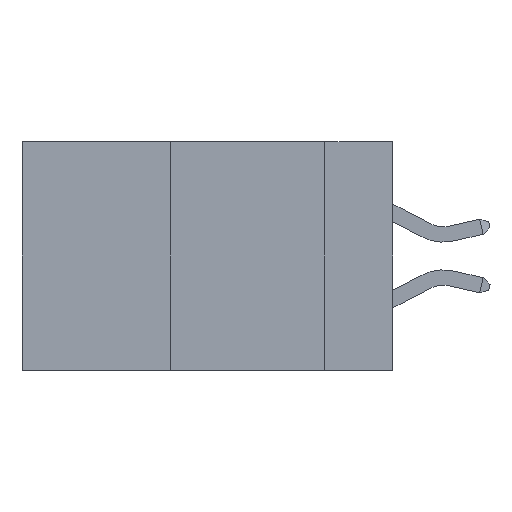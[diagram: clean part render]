
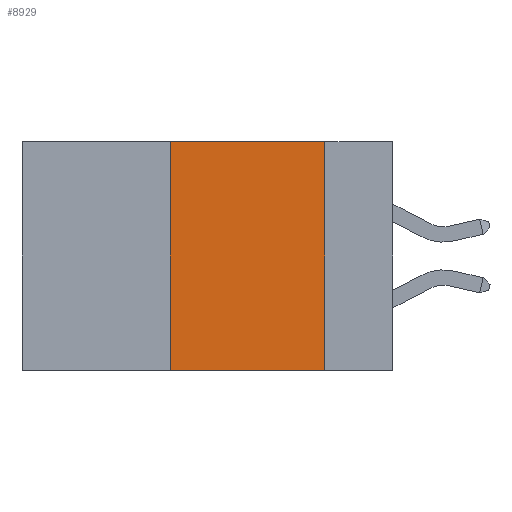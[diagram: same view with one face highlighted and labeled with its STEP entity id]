
A CAD part, left-side view. The second image highlights one B-rep face of the part: STEP entity #8929.
In plain terms, the highlighted planar face has unit normal (-1, 0, 0).
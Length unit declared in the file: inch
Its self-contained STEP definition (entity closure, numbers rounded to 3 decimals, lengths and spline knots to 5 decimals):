
#153 = VECTOR ( 'NONE', #24012, 39.37008 ) ;
#1043 = CARTESIAN_POINT ( 'NONE',  ( 0., 0.36, -0.37 ) ) ;
#1958 = CARTESIAN_POINT ( 'NONE',  ( 0., 0.36, 0. ) ) ;
#2331 = VERTEX_POINT ( 'NONE', #15774 ) ;
#4583 = ORIENTED_EDGE ( 'NONE', *, *, #18128, .F. ) ;
#4598 = LINE ( 'NONE', #14453, #153 ) ;
#5379 = DIRECTION ( 'NONE',  ( 1., 0., 0. ) ) ;
#6328 = LINE ( 'NONE', #19755, #18650 ) ;
#7179 = CARTESIAN_POINT ( 'NONE',  ( 0., 0.6, 0. ) ) ;
#8027 = EDGE_LOOP ( 'NONE', ( #4583, #11248, #17220, #20234 ) ) ;
#8929 = ADVANCED_FACE ( 'NONE', ( #18200 ), #22110, .F. ) ;
#8954 = VECTOR ( 'NONE', #24085, 39.37008 ) ;
#9553 = VERTEX_POINT ( 'NONE', #16440 ) ;
#10138 = EDGE_CURVE ( 'NONE', #13651, #17912, #16940, .T. ) ;
#10713 = EDGE_CURVE ( 'NONE', #17912, #9553, #4598, .T. ) ;
#10892 = CARTESIAN_POINT ( 'NONE',  ( 0., 0.6, -0.37 ) ) ;
#11248 = ORIENTED_EDGE ( 'NONE', *, *, #10713, .F. ) ;
#13651 = VERTEX_POINT ( 'NONE', #1043 ) ;
#14453 = CARTESIAN_POINT ( 'NONE',  ( 0., 0.6, 0. ) ) ;
#15774 = CARTESIAN_POINT ( 'NONE',  ( 0., 0.11, -0.37 ) ) ;
#16440 = CARTESIAN_POINT ( 'NONE',  ( 0., 0.11, 0. ) ) ;
#16940 = LINE ( 'NONE', #1958, #18092 ) ;
#17220 = ORIENTED_EDGE ( 'NONE', *, *, #10138, .F. ) ;
#17912 = VERTEX_POINT ( 'NONE', #23329 ) ;
#18092 = VECTOR ( 'NONE', #24131, 39.37008 ) ;
#18128 = EDGE_CURVE ( 'NONE', #9553, #2331, #6328, .T. ) ;
#18200 = FACE_OUTER_BOUND ( 'NONE', #8027, .T. ) ;
#18481 = DIRECTION ( 'NONE',  ( 0., 0., -1. ) ) ;
#18650 = VECTOR ( 'NONE', #21778, 39.37008 ) ;
#19755 = CARTESIAN_POINT ( 'NONE',  ( 0., 0.11, 0. ) ) ;
#20045 = AXIS2_PLACEMENT_3D ( 'NONE', #7179, #5379, #18481 ) ;
#20234 = ORIENTED_EDGE ( 'NONE', *, *, #22629, .T. ) ;
#21778 = DIRECTION ( 'NONE',  ( 0., 0., -1. ) ) ;
#21821 = LINE ( 'NONE', #10892, #8954 ) ;
#22110 = PLANE ( 'NONE',  #20045 ) ;
#22629 = EDGE_CURVE ( 'NONE', #13651, #2331, #21821, .T. ) ;
#23329 = CARTESIAN_POINT ( 'NONE',  ( 0., 0.36, 0. ) ) ;
#24012 = DIRECTION ( 'NONE',  ( 0., -1., 0. ) ) ;
#24085 = DIRECTION ( 'NONE',  ( 0., -1., 0. ) ) ;
#24131 = DIRECTION ( 'NONE',  ( 0., 0., 1. ) ) ;
